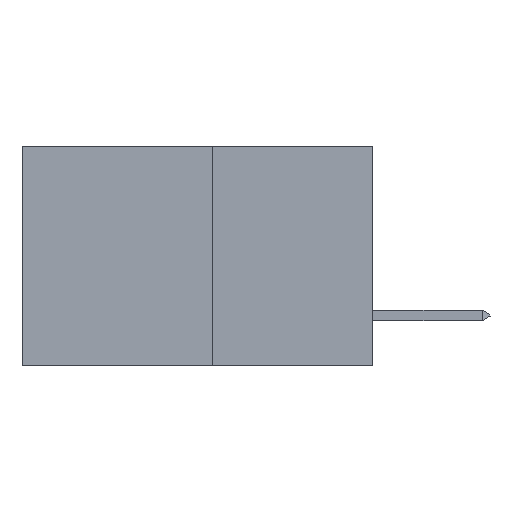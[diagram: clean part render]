
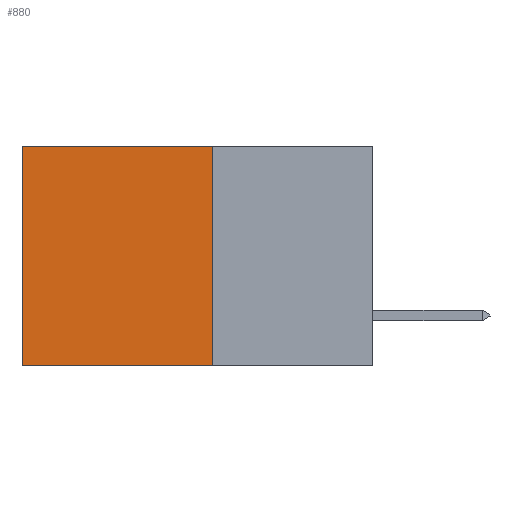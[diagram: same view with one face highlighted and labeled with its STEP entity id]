
A CAD part, left-side view. The second image highlights one B-rep face of the part: STEP entity #880.
In plain terms, the highlighted planar face has unit normal (-1, 0, 0).
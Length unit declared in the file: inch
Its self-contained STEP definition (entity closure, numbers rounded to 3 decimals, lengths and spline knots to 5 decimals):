
#460 = EDGE_CURVE ( 'NONE', #19691, #18976, #20021, .T. ) ;
#880 = ADVANCED_FACE ( 'NONE', ( #20659 ), #9255, .F. ) ;
#2818 = CARTESIAN_POINT ( 'NONE',  ( 0.277, 0.27, -0.37 ) ) ;
#3615 = ORIENTED_EDGE ( 'NONE', *, *, #10530, .F. ) ;
#4106 = LINE ( 'NONE', #21736, #24617 ) ;
#4555 = DIRECTION ( 'NONE',  ( 0., 1., 0. ) ) ;
#4951 = CARTESIAN_POINT ( 'NONE',  ( 0.277, 0.27, -0.37 ) ) ;
#5811 = VERTEX_POINT ( 'NONE', #22498 ) ;
#6063 = ORIENTED_EDGE ( 'NONE', *, *, #15406, .T. ) ;
#6144 = EDGE_CURVE ( 'NONE', #5811, #24851, #27796, .T. ) ;
#6523 = LINE ( 'NONE', #6725, #16336 ) ;
#6725 = CARTESIAN_POINT ( 'NONE',  ( 0.277, 0.27, -0.37 ) ) ;
#7883 = CARTESIAN_POINT ( 'NONE',  ( 0.277, 0.27, 0. ) ) ;
#9255 = PLANE ( 'NONE',  #21794 ) ;
#10475 = CARTESIAN_POINT ( 'NONE',  ( 0.277, 0.27, -0.37 ) ) ;
#10530 = EDGE_CURVE ( 'NONE', #5811, #19691, #6523, .T. ) ;
#11172 = ORIENTED_EDGE ( 'NONE', *, *, #6144, .T. ) ;
#14771 = CARTESIAN_POINT ( 'NONE',  ( 0.277, 0.59, 0. ) ) ;
#15406 = EDGE_CURVE ( 'NONE', #24851, #18976, #4106, .T. ) ;
#16336 = VECTOR ( 'NONE', #19892, 39.37008 ) ;
#17498 = EDGE_LOOP ( 'NONE', ( #6063, #20727, #3615, #11172 ) ) ;
#18976 = VERTEX_POINT ( 'NONE', #27070 ) ;
#19648 = DIRECTION ( 'NONE',  ( 0., 0., -1. ) ) ;
#19691 = VERTEX_POINT ( 'NONE', #10475 ) ;
#19892 = DIRECTION ( 'NONE',  ( 0., 0., -1. ) ) ;
#20021 = LINE ( 'NONE', #4951, #20687 ) ;
#20206 = DIRECTION ( 'NONE',  ( 0., 0., -1. ) ) ;
#20241 = DIRECTION ( 'NONE',  ( 1., 0., 0. ) ) ;
#20659 = FACE_OUTER_BOUND ( 'NONE', #17498, .T. ) ;
#20687 = VECTOR ( 'NONE', #4555, 39.37008 ) ;
#20727 = ORIENTED_EDGE ( 'NONE', *, *, #460, .F. ) ;
#21736 = CARTESIAN_POINT ( 'NONE',  ( 0.277, 0.59, -0.37 ) ) ;
#21794 = AXIS2_PLACEMENT_3D ( 'NONE', #2818, #20241, #20206 ) ;
#22498 = CARTESIAN_POINT ( 'NONE',  ( 0.277, 0.27, 0. ) ) ;
#24617 = VECTOR ( 'NONE', #19648, 39.37008 ) ;
#24851 = VERTEX_POINT ( 'NONE', #14771 ) ;
#27070 = CARTESIAN_POINT ( 'NONE',  ( 0.277, 0.59, -0.37 ) ) ;
#27120 = VECTOR ( 'NONE', #27491, 39.37008 ) ;
#27491 = DIRECTION ( 'NONE',  ( 0., 1., 0. ) ) ;
#27796 = LINE ( 'NONE', #7883, #27120 ) ;
